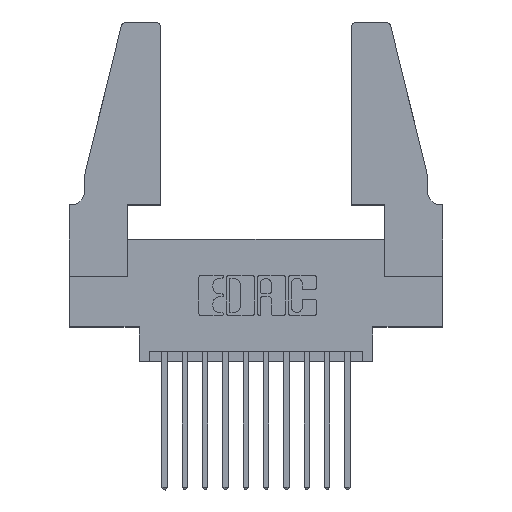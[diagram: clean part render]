
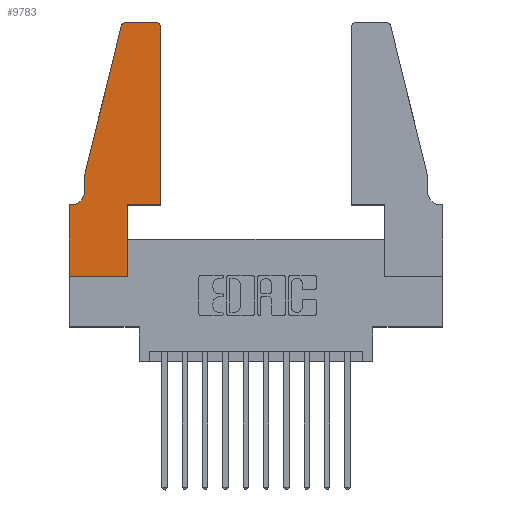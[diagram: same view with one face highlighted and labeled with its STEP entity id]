
A CAD part, top view. The second image highlights one B-rep face of the part: STEP entity #9783.
In plain terms, the highlighted planar face has unit normal (0, 0, 1).
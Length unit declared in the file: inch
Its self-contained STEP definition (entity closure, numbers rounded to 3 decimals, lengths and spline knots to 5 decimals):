
#326 = DIRECTION ( 'NONE',  ( 0., 0., 1. ) ) ;
#335 = VERTEX_POINT ( 'NONE', #13515 ) ;
#431 = LINE ( 'NONE', #7596, #3623 ) ;
#463 = CARTESIAN_POINT ( 'NONE',  ( 0., 0.35, 0.37 ) ) ;
#647 = DIRECTION ( 'NONE',  ( 1., 0., 0. ) ) ;
#1097 = VERTEX_POINT ( 'NONE', #13358 ) ;
#1251 = VERTEX_POINT ( 'NONE', #5700 ) ;
#1545 = VECTOR ( 'NONE', #1876, 39.37008 ) ;
#1775 = FACE_OUTER_BOUND ( 'NONE', #8873, .T. ) ;
#1876 = DIRECTION ( 'NONE',  ( -1., 0., 0. ) ) ;
#1896 = VECTOR ( 'NONE', #14487, 39.37008 ) ;
#1990 = VERTEX_POINT ( 'NONE', #9750 ) ;
#2008 = EDGE_CURVE ( 'NONE', #3155, #5715, #11473, .T. ) ;
#2033 = ORIENTED_EDGE ( 'NONE', *, *, #11749, .T. ) ;
#2217 = CARTESIAN_POINT ( 'NONE',  ( 0.0055, 0.42, 0.37 ) ) ;
#2358 = CARTESIAN_POINT ( 'NONE',  ( 0.25487, 1.22718, 0.37 ) ) ;
#2647 = DIRECTION ( 'NONE',  ( 0., 1., 0. ) ) ;
#2665 = EDGE_CURVE ( 'NONE', #6018, #5827, #10615, .T. ) ;
#2982 = EDGE_CURVE ( 'NONE', #12628, #1251, #431, .T. ) ;
#3055 = CARTESIAN_POINT ( 'NONE',  ( 0.0755, 0.35, 0.37 ) ) ;
#3063 = ORIENTED_EDGE ( 'NONE', *, *, #5029, .T. ) ;
#3155 = VERTEX_POINT ( 'NONE', #6973 ) ;
#3173 = LINE ( 'NONE', #11185, #1896 ) ;
#3309 = VECTOR ( 'NONE', #8487, 39.37008 ) ;
#3375 = CIRCLE ( 'NONE', #11762, 0.07 ) ;
#3505 = EDGE_CURVE ( 'NONE', #3964, #3155, #14053, .T. ) ;
#3586 = VERTEX_POINT ( 'NONE', #6639 ) ;
#3623 = VECTOR ( 'NONE', #6601, 39.37008 ) ;
#3762 = ORIENTED_EDGE ( 'NONE', *, *, #14214, .T. ) ;
#3891 = ORIENTED_EDGE ( 'NONE', *, *, #14396, .T. ) ;
#3964 = VERTEX_POINT ( 'NONE', #6704 ) ;
#4001 = VECTOR ( 'NONE', #13810, 39.37008 ) ;
#4052 = EDGE_CURVE ( 'NONE', #1097, #3586, #4126, .T. ) ;
#4126 = CIRCLE ( 'NONE', #4841, 0.03 ) ;
#4203 = CARTESIAN_POINT ( 'NONE',  ( 0.0755, 0.5, 0.37 ) ) ;
#4841 = AXIS2_PLACEMENT_3D ( 'NONE', #4977, #326, #5828 ) ;
#4915 = DIRECTION ( 'NONE',  ( 0., 0., 1. ) ) ;
#4963 = CARTESIAN_POINT ( 'NONE',  ( 0., 0., 0.37 ) ) ;
#4977 = CARTESIAN_POINT ( 'NONE',  ( 0.4205, 1.22, 0.37 ) ) ;
#5029 = EDGE_CURVE ( 'NONE', #1990, #3964, #3375, .T. ) ;
#5053 = LINE ( 'NONE', #13190, #7308 ) ;
#5137 = DIRECTION ( 'NONE',  ( 0., 0., 1. ) ) ;
#5397 = CARTESIAN_POINT ( 'NONE',  ( 0.284, 1.25, 0.37 ) ) ;
#5700 = CARTESIAN_POINT ( 'NONE',  ( 0.2865, 0.35, 0.37 ) ) ;
#5715 = VERTEX_POINT ( 'NONE', #10258 ) ;
#5827 = VERTEX_POINT ( 'NONE', #2358 ) ;
#5828 = DIRECTION ( 'NONE',  ( 1., 0., 0. ) ) ;
#5877 = CARTESIAN_POINT ( 'NONE',  ( 0.0755, 0.5, 0.37 ) ) ;
#6016 = CARTESIAN_POINT ( 'NONE',  ( 0.2865, 0., 0.37 ) ) ;
#6018 = VERTEX_POINT ( 'NONE', #5397 ) ;
#6020 = AXIS2_PLACEMENT_3D ( 'NONE', #9680, #5137, #647 ) ;
#6052 = ORIENTED_EDGE ( 'NONE', *, *, #7185, .T. ) ;
#6262 = CARTESIAN_POINT ( 'NONE',  ( 0.2605, 1.25, 0.37 ) ) ;
#6281 = LINE ( 'NONE', #6262, #1545 ) ;
#6380 = LINE ( 'NONE', #8422, #11658 ) ;
#6530 = EDGE_CURVE ( 'NONE', #335, #1097, #10652, .T. ) ;
#6601 = DIRECTION ( 'NONE',  ( 0., 1., 0. ) ) ;
#6639 = CARTESIAN_POINT ( 'NONE',  ( 0.4205, 1.25, 0.37 ) ) ;
#6704 = CARTESIAN_POINT ( 'NONE',  ( 0.0055, 0.35, 0.37 ) ) ;
#6973 = CARTESIAN_POINT ( 'NONE',  ( 0., 0.35, 0.37 ) ) ;
#7185 = EDGE_CURVE ( 'NONE', #9462, #1990, #10469, .T. ) ;
#7308 = VECTOR ( 'NONE', #14322, 39.37008 ) ;
#7515 = ORIENTED_EDGE ( 'NONE', *, *, #2665, .T. ) ;
#7596 = CARTESIAN_POINT ( 'NONE',  ( 0.2865, 0.35, 0.37 ) ) ;
#7843 = AXIS2_PLACEMENT_3D ( 'NONE', #463, #4915, #8323 ) ;
#8114 = ORIENTED_EDGE ( 'NONE', *, *, #4052, .T. ) ;
#8323 = DIRECTION ( 'NONE',  ( 1., 0., 0. ) ) ;
#8422 = CARTESIAN_POINT ( 'NONE',  ( 0.0755, 0.5, 0.37 ) ) ;
#8487 = DIRECTION ( 'NONE',  ( 0., -1., 0. ) ) ;
#8873 = EDGE_LOOP ( 'NONE', ( #9968, #7515, #3762, #6052, #3063, #10260, #14424, #2033, #9855, #3891, #11819, #8114 ) ) ;
#9462 = VERTEX_POINT ( 'NONE', #4203 ) ;
#9599 = DIRECTION ( 'NONE',  ( -0.239, -0.971, 0. ) ) ;
#9680 = CARTESIAN_POINT ( 'NONE',  ( 0.284, 1.22, 0.37 ) ) ;
#9750 = CARTESIAN_POINT ( 'NONE',  ( 0.0755, 0.42, 0.37 ) ) ;
#9783 = ADVANCED_FACE ( 'NONE', ( #1775 ), #13956, .T. ) ;
#9802 = DIRECTION ( 'NONE',  ( -1., 0., 0. ) ) ;
#9855 = ORIENTED_EDGE ( 'NONE', *, *, #2982, .T. ) ;
#9967 = VECTOR ( 'NONE', #2647, 39.37008 ) ;
#9968 = ORIENTED_EDGE ( 'NONE', *, *, #12151, .T. ) ;
#10139 = DIRECTION ( 'NONE',  ( 0., 0., -1. ) ) ;
#10258 = CARTESIAN_POINT ( 'NONE',  ( 0., 0., 0.37 ) ) ;
#10260 = ORIENTED_EDGE ( 'NONE', *, *, #3505, .T. ) ;
#10469 = LINE ( 'NONE', #5877, #3309 ) ;
#10615 = CIRCLE ( 'NONE', #6020, 0.03 ) ;
#10652 = LINE ( 'NONE', #11643, #9967 ) ;
#11185 = CARTESIAN_POINT ( 'NONE',  ( 0., 0., 0.37 ) ) ;
#11473 = LINE ( 'NONE', #4963, #4001 ) ;
#11643 = CARTESIAN_POINT ( 'NONE',  ( 0.4505, 0.35, 0.37 ) ) ;
#11658 = VECTOR ( 'NONE', #9599, 39.37008 ) ;
#11749 = EDGE_CURVE ( 'NONE', #5715, #12628, #3173, .T. ) ;
#11762 = AXIS2_PLACEMENT_3D ( 'NONE', #2217, #10139, #12155 ) ;
#11819 = ORIENTED_EDGE ( 'NONE', *, *, #6530, .T. ) ;
#12151 = EDGE_CURVE ( 'NONE', #3586, #6018, #6281, .T. ) ;
#12155 = DIRECTION ( 'NONE',  ( -1., 0., 0. ) ) ;
#12628 = VERTEX_POINT ( 'NONE', #6016 ) ;
#13190 = CARTESIAN_POINT ( 'NONE',  ( 0.4505, 0.35, 0.37 ) ) ;
#13358 = CARTESIAN_POINT ( 'NONE',  ( 0.4505, 1.22, 0.37 ) ) ;
#13515 = CARTESIAN_POINT ( 'NONE',  ( 0.4505, 0.35, 0.37 ) ) ;
#13810 = DIRECTION ( 'NONE',  ( 0., -1., 0. ) ) ;
#13871 = VECTOR ( 'NONE', #9802, 39.37008 ) ;
#13956 = PLANE ( 'NONE',  #7843 ) ;
#14053 = LINE ( 'NONE', #3055, #13871 ) ;
#14214 = EDGE_CURVE ( 'NONE', #5827, #9462, #6380, .T. ) ;
#14322 = DIRECTION ( 'NONE',  ( 1., 0., 0. ) ) ;
#14396 = EDGE_CURVE ( 'NONE', #1251, #335, #5053, .T. ) ;
#14424 = ORIENTED_EDGE ( 'NONE', *, *, #2008, .T. ) ;
#14487 = DIRECTION ( 'NONE',  ( 1., 0., 0. ) ) ;
